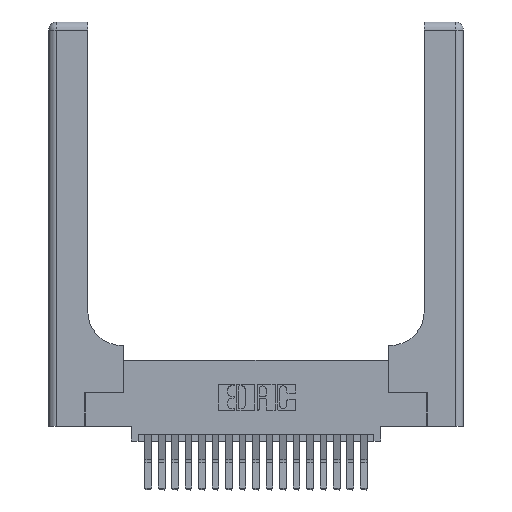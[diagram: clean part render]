
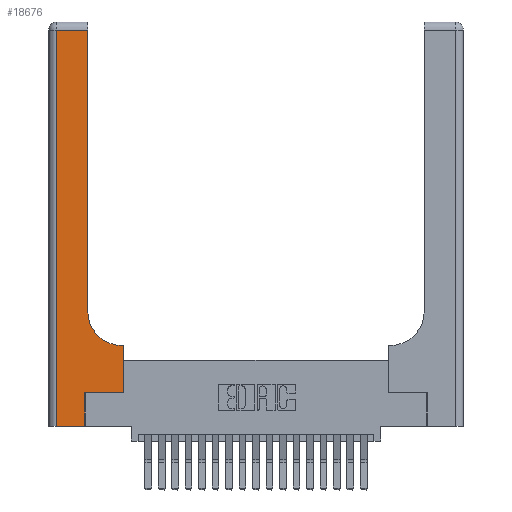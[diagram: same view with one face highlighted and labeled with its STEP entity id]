
A CAD part, top view. The second image highlights one B-rep face of the part: STEP entity #18676.
In plain terms, the highlighted planar face has unit normal (0, 0, 1).
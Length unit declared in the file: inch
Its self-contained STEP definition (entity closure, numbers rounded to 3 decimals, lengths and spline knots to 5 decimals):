
#182 = CARTESIAN_POINT ( 'NONE',  ( 0.5585, 0.25, 0.37 ) ) ;
#457 = DIRECTION ( 'NONE',  ( 1., 0., 0. ) ) ;
#763 = CARTESIAN_POINT ( 'NONE',  ( 0.06, 2.94, 0.37 ) ) ;
#844 = EDGE_CURVE ( 'NONE', #9610, #8078, #16199, .T. ) ;
#1390 = LINE ( 'NONE', #15982, #14695 ) ;
#1420 = EDGE_CURVE ( 'NONE', #3132, #17039, #15695, .T. ) ;
#1623 = VECTOR ( 'NONE', #12504, 39.37008 ) ;
#2042 = DIRECTION ( 'NONE',  ( 0., 1., 0. ) ) ;
#2044 = VECTOR ( 'NONE', #2042, 39.37008 ) ;
#2173 = CARTESIAN_POINT ( 'NONE',  ( 0., 3., 0.37 ) ) ;
#2392 = VERTEX_POINT ( 'NONE', #14245 ) ;
#2619 = CARTESIAN_POINT ( 'NONE',  ( 0.5415, 0.85, 0.37 ) ) ;
#3132 = VERTEX_POINT ( 'NONE', #18175 ) ;
#3741 = LINE ( 'NONE', #13173, #16778 ) ;
#4020 = DIRECTION ( 'NONE',  ( -1., 0., 0. ) ) ;
#4451 = DIRECTION ( 'NONE',  ( 1., 0., 0. ) ) ;
#4594 = DIRECTION ( 'NONE',  ( -1., 0., 0. ) ) ;
#4703 = CARTESIAN_POINT ( 'NONE',  ( 0.269, 0., 0.37 ) ) ;
#6324 = CARTESIAN_POINT ( 'NONE',  ( 0.269, 0.25, 0.37 ) ) ;
#6399 = VERTEX_POINT ( 'NONE', #18444 ) ;
#6676 = VECTOR ( 'NONE', #16103, 39.37008 ) ;
#6787 = EDGE_CURVE ( 'NONE', #17039, #6399, #12105, .T. ) ;
#7044 = ORIENTED_EDGE ( 'NONE', *, *, #13159, .T. ) ;
#7068 = ORIENTED_EDGE ( 'NONE', *, *, #6787, .T. ) ;
#7263 = EDGE_CURVE ( 'NONE', #6399, #2392, #11348, .T. ) ;
#7474 = VERTEX_POINT ( 'NONE', #763 ) ;
#8078 = VERTEX_POINT ( 'NONE', #6324 ) ;
#8129 = CARTESIAN_POINT ( 'NONE',  ( 0.269, 0., 0.37 ) ) ;
#9016 = VERTEX_POINT ( 'NONE', #13303 ) ;
#9172 = DIRECTION ( 'NONE',  ( 1., 0., 0. ) ) ;
#9610 = VERTEX_POINT ( 'NONE', #4703 ) ;
#9664 = CARTESIAN_POINT ( 'NONE',  ( 0.06, 3., 0.37 ) ) ;
#10828 = CARTESIAN_POINT ( 'NONE',  ( 0.5415, 0.6, 0.37 ) ) ;
#10991 = ORIENTED_EDGE ( 'NONE', *, *, #844, .T. ) ;
#11348 = LINE ( 'NONE', #12485, #2044 ) ;
#11775 = VECTOR ( 'NONE', #16387, 39.37008 ) ;
#12011 = EDGE_CURVE ( 'NONE', #8078, #14042, #1390, .T. ) ;
#12105 = CIRCLE ( 'NONE', #21916, 0.25 ) ;
#12485 = CARTESIAN_POINT ( 'NONE',  ( 0.2915, 3., 0.37 ) ) ;
#12504 = DIRECTION ( 'NONE',  ( 0., 1., 0. ) ) ;
#12920 = LINE ( 'NONE', #19166, #20644 ) ;
#13159 = EDGE_CURVE ( 'NONE', #14042, #3132, #15438, .T. ) ;
#13173 = CARTESIAN_POINT ( 'NONE',  ( 0., 2.94, 0.37 ) ) ;
#13303 = CARTESIAN_POINT ( 'NONE',  ( 0.06, 0., 0.37 ) ) ;
#13383 = AXIS2_PLACEMENT_3D ( 'NONE', #2173, #14329, #4020 ) ;
#13446 = CARTESIAN_POINT ( 'NONE',  ( 0.5585, 0.25, 0.37 ) ) ;
#14042 = VERTEX_POINT ( 'NONE', #13446 ) ;
#14245 = CARTESIAN_POINT ( 'NONE',  ( 0.2915, 2.94, 0.37 ) ) ;
#14250 = ORIENTED_EDGE ( 'NONE', *, *, #1420, .T. ) ;
#14329 = DIRECTION ( 'NONE',  ( 0., 0., -1. ) ) ;
#14352 = EDGE_CURVE ( 'NONE', #9016, #9610, #12920, .T. ) ;
#14695 = VECTOR ( 'NONE', #457, 39.37008 ) ;
#14706 = DIRECTION ( 'NONE',  ( 0., 0., -1. ) ) ;
#14820 = FACE_OUTER_BOUND ( 'NONE', #16015, .T. ) ;
#15438 = LINE ( 'NONE', #182, #1623 ) ;
#15695 = LINE ( 'NONE', #16233, #6676 ) ;
#15982 = CARTESIAN_POINT ( 'NONE',  ( 0.269, 0.25, 0.37 ) ) ;
#16015 = EDGE_LOOP ( 'NONE', ( #18491, #19783, #18505, #17232, #10991, #18525, #7044, #14250, #7068 ) ) ;
#16103 = DIRECTION ( 'NONE',  ( -1., 0., 0. ) ) ;
#16199 = LINE ( 'NONE', #8129, #11775 ) ;
#16233 = CARTESIAN_POINT ( 'NONE',  ( 0.2915, 0.6, 0.37 ) ) ;
#16387 = DIRECTION ( 'NONE',  ( 0., 1., 0. ) ) ;
#16778 = VECTOR ( 'NONE', #4594, 39.37008 ) ;
#16822 = LINE ( 'NONE', #9664, #17338 ) ;
#17039 = VERTEX_POINT ( 'NONE', #10828 ) ;
#17232 = ORIENTED_EDGE ( 'NONE', *, *, #14352, .T. ) ;
#17338 = VECTOR ( 'NONE', #19650, 39.37008 ) ;
#17522 = PLANE ( 'NONE',  #13383 ) ;
#18175 = CARTESIAN_POINT ( 'NONE',  ( 0.5585, 0.6, 0.37 ) ) ;
#18444 = CARTESIAN_POINT ( 'NONE',  ( 0.2915, 0.85, 0.37 ) ) ;
#18491 = ORIENTED_EDGE ( 'NONE', *, *, #7263, .T. ) ;
#18505 = ORIENTED_EDGE ( 'NONE', *, *, #19474, .T. ) ;
#18525 = ORIENTED_EDGE ( 'NONE', *, *, #12011, .T. ) ;
#18676 = ADVANCED_FACE ( 'NONE', ( #14820 ), #17522, .F. ) ;
#19166 = CARTESIAN_POINT ( 'NONE',  ( 0., 0., 0.37 ) ) ;
#19474 = EDGE_CURVE ( 'NONE', #7474, #9016, #16822, .T. ) ;
#19650 = DIRECTION ( 'NONE',  ( 0., -1., 0. ) ) ;
#19783 = ORIENTED_EDGE ( 'NONE', *, *, #20147, .T. ) ;
#20147 = EDGE_CURVE ( 'NONE', #2392, #7474, #3741, .T. ) ;
#20644 = VECTOR ( 'NONE', #9172, 39.37008 ) ;
#21916 = AXIS2_PLACEMENT_3D ( 'NONE', #2619, #14706, #4451 ) ;
